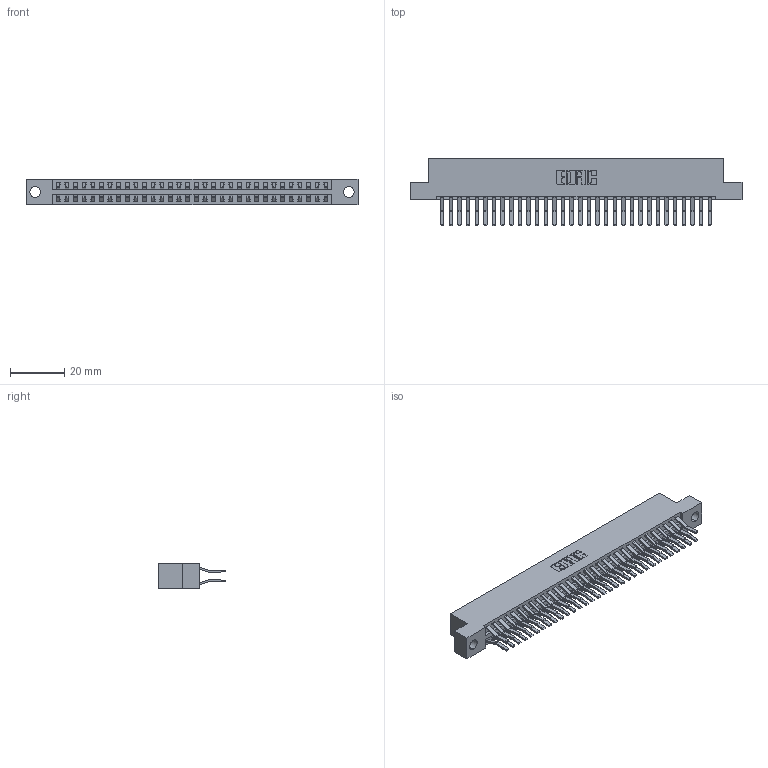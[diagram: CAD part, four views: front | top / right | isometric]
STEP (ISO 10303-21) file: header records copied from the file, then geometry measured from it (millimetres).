
FILE_DESCRIPTION (( 'STEP AP203' ), '1' );
FILE_NAME ('396-064-560-204.STEP', '2019-10-30T17:58:30', ( '' ), ( '' ), 'SwSTEP 2.0', 'SolidWorks 2016', '' );
FILE_SCHEMA (( 'CONFIG_CONTROL_DESIGN' ));
Length unit declared in the file: inch
Products named in the file (3): 346 Part_Flush Mounting Lugs - 0.156 Dia-TH; 396-064-560-204; 345-292-001_560 Tail
Assembly tree (65 placements, depth 2):
  396-064-560-204
    346 Part_Flush Mounting Lugs - 0.156 Dia-TH
    345-292-001_560 Tail  x64
Bounding box: 122.17 x 24.78 x 9.4 mm (x, y, z)
Volume: 12167.5 mm3; surface area: 17500.3 mm2
Topology: 65 solids, 65 shells, 3578 faces, 10633 edges, 7002 vertices
Faces by surface type: plane 2316, cylinder 1262
Entity records: 22321 total; most frequent: CARTESIAN_POINT 3692, ORIENTED_EDGE 3626, DIRECTION 3309, EDGE_CURVE 1813, VECTOR 1549, LINE 1549, VERTEX_POINT 1206, AXIS2_PLACEMENT_3D 880
